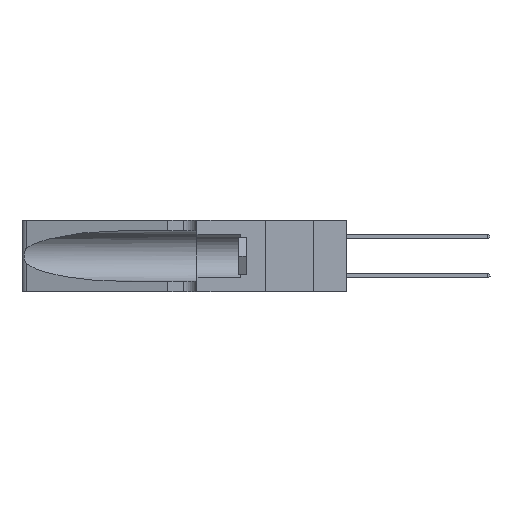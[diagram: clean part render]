
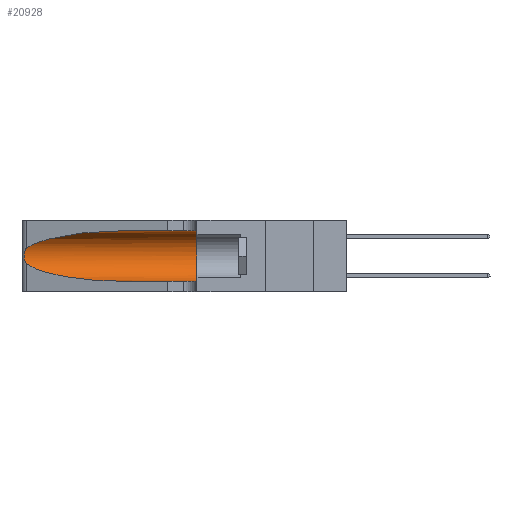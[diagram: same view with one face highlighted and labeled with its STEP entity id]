
A CAD part, left-side view. The second image highlights one B-rep face of the part: STEP entity #20928.
In plain terms, the highlighted cylindrical face has radius 3.308 mm (diameter 6.617 mm), a partial arc.
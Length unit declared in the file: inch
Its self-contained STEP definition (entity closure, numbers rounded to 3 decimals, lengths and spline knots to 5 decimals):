
#522 = VECTOR ( 'NONE', #25602, 39.37008 ) ;
#565 = AXIS2_PLACEMENT_3D ( 'NONE', #19608, #23783, #10734 ) ;
#960 = EDGE_CURVE ( 'NONE', #8144, #22175, #27132, .T. ) ;
#1241 = ORIENTED_EDGE ( 'NONE', *, *, #960, .T. ) ;
#1690 = VERTEX_POINT ( 'NONE', #23200 ) ;
#2027 = EDGE_LOOP ( 'NONE', ( #1241, #18153, #17085, #13312, #13359, #27412 ) ) ;
#2455 = EDGE_CURVE ( 'NONE', #8144, #1690, #9759, .T. ) ;
#3530 = EDGE_CURVE ( 'NONE', #1690, #6931, #11722, .T. ) ;
#3844 = DIRECTION ( 'NONE',  ( 0., 1., 0. ) ) ;
#4071 = CARTESIAN_POINT ( 'NONE',  ( 0.25487, 1.22718, 0.14631 ) ) ;
#4988 = FACE_OUTER_BOUND ( 'NONE', #2027, .T. ) ;
#5533 = CARTESIAN_POINT ( 'NONE',  ( 0.1305, 0.72297, 0.05475 ) ) ;
#6007 = CARTESIAN_POINT ( 'NONE',  ( 0.25854, 1.2359, 0.20912 ) ) ;
#6095 = CARTESIAN_POINT ( 'NONE',  ( 0.25639, 1.23184, 0.21858 ) ) ;
#6526 = CARTESIAN_POINT ( 'NONE',  ( 0.18966, 0.96281, 0.31525 ) ) ;
#6889 = VECTOR ( 'NONE', #8099, 39.37008 ) ;
#6931 = VERTEX_POINT ( 'NONE', #20959 ) ;
#7539 = CARTESIAN_POINT ( 'NONE',  ( 0.18966, 0.96281, 0.05475 ) ) ;
#8099 = DIRECTION ( 'NONE',  ( 0., -1., 0. ) ) ;
#8144 = VERTEX_POINT ( 'NONE', #23531 ) ;
#8605 = CARTESIAN_POINT ( 'NONE',  ( 0.26075, 1.23896, 0.19203 ) ) ;
#8644 = CARTESIAN_POINT ( 'NONE',  ( 0.25487, 1.22718, 0.14631 ) ) ;
#9153 = CARTESIAN_POINT ( 'NONE',  ( 0.25789, 1.23486, 0.15765 ) ) ;
#9521 = CARTESIAN_POINT ( 'NONE',  ( 0.2373, 1.15595, 0.08982 ) ) ;
#9759 = LINE ( 'NONE', #17137, #522 ) ;
#9943 = CARTESIAN_POINT ( 'NONE',  ( 0.25555, 1.22994, 0.2215 ) ) ;
#10236 = CARTESIAN_POINT ( 'NONE',  ( 0.26018, 1.23835, 0.19895 ) ) ;
#10396 = EDGE_CURVE ( 'NONE', #22175, #27143, #17878, .T. ) ;
#10734 = DIRECTION ( 'NONE',  ( 0., 0., -1. ) ) ;
#11075 = CARTESIAN_POINT ( 'NONE',  ( 0.26075, 1.23896, 0.178 ) ) ;
#11722 = CIRCLE ( 'NONE', #22953, 0.13025 ) ;
#13095 = CARTESIAN_POINT ( 'NONE',  ( 0.1305, 0.72297, 0.31525 ) ) ;
#13187 = CARTESIAN_POINT ( 'NONE',  ( 0.25487, 1.22718, 0.22369 ) ) ;
#13312 = ORIENTED_EDGE ( 'NONE', *, *, #27218, .T. ) ;
#13359 = ORIENTED_EDGE ( 'NONE', *, *, #3530, .F. ) ;
#13746 = EDGE_CURVE ( 'NONE', #27143, #21360, #19648, .T. ) ;
#14034 = CARTESIAN_POINT ( 'NONE',  ( 0.25487, 1.22718, 0.14631 ) ) ;
#15866 = CARTESIAN_POINT ( 'NONE',  ( 0.25487, 1.22718, 0.22369 ) ) ;
#16587 = CYLINDRICAL_SURFACE ( 'NONE', #565, 0.13025 ) ;
#17085 = ORIENTED_EDGE ( 'NONE', *, *, #13746, .T. ) ;
#17137 = CARTESIAN_POINT ( 'NONE',  ( 0.1305, 1.61858, 0.31525 ) ) ;
#17368 = CARTESIAN_POINT ( 'NONE',  ( 0.2373, 1.15595, 0.28018 ) ) ;
#17478 = CARTESIAN_POINT ( 'NONE',  ( 0.25639, 1.23186, 0.15144 ) ) ;
#17878 = B_SPLINE_CURVE_WITH_KNOTS ( 'NONE', 3,
 ( #26562, #9943, #6095, #23300, #6007, #10236, #8605, #11075, #27424, #23155, #9153, #17478, #21593, #8644 ),
 .UNSPECIFIED., .F., .F.,
 ( 4, 2, 2, 2, 2, 2, 4 ),
 ( 0., 0.00027, 0.00053, 0.00107, 0.0016, 0.00187, 0.00214 ),
 .UNSPECIFIED. ) ;
#18153 = ORIENTED_EDGE ( 'NONE', *, *, #10396, .T. ) ;
#19608 = CARTESIAN_POINT ( 'NONE',  ( 0.1305, 1.61858, 0.185 ) ) ;
#19648 =( BOUNDED_CURVE ( )  B_SPLINE_CURVE ( 3, ( #14034, #9521, #7539, #27119 ),
 .UNSPECIFIED., .F., .F. ) 
 B_SPLINE_CURVE_WITH_KNOTS ( ( 4, 4 ),
 ( 3.44316, 4.71239 ),
 .UNSPECIFIED. ) 
 CURVE ( )  GEOMETRIC_REPRESENTATION_ITEM ( )  RATIONAL_B_SPLINE_CURVE ( ( 1., 0.87, 0.87, 1. ) ) 
 REPRESENTATION_ITEM ( '' )  );
#20928 = ADVANCED_FACE ( 'NONE', ( #4988 ), #16587, .F. ) ;
#20959 = CARTESIAN_POINT ( 'NONE',  ( 0.1305, 0.35, 0.05475 ) ) ;
#21360 = VERTEX_POINT ( 'NONE', #5533 ) ;
#21386 = CARTESIAN_POINT ( 'NONE',  ( 0.1305, 0.35, 0.185 ) ) ;
#21593 = CARTESIAN_POINT ( 'NONE',  ( 0.25555, 1.22993, 0.14849 ) ) ;
#22175 = VERTEX_POINT ( 'NONE', #15866 ) ;
#22953 = AXIS2_PLACEMENT_3D ( 'NONE', #21386, #3844, #23568 ) ;
#23155 = CARTESIAN_POINT ( 'NONE',  ( 0.25856, 1.23593, 0.16098 ) ) ;
#23200 = CARTESIAN_POINT ( 'NONE',  ( 0.1305, 0.35, 0.31525 ) ) ;
#23300 = CARTESIAN_POINT ( 'NONE',  ( 0.25787, 1.23484, 0.2124 ) ) ;
#23531 = CARTESIAN_POINT ( 'NONE',  ( 0.1305, 0.72297, 0.31525 ) ) ;
#23568 = DIRECTION ( 'NONE',  ( 0., 0., 1. ) ) ;
#23783 = DIRECTION ( 'NONE',  ( 0., -1., 0. ) ) ;
#25394 = CARTESIAN_POINT ( 'NONE',  ( 0.1305, 1.61858, 0.05475 ) ) ;
#25602 = DIRECTION ( 'NONE',  ( 0., -1., 0. ) ) ;
#25947 = LINE ( 'NONE', #25394, #6889 ) ;
#26562 = CARTESIAN_POINT ( 'NONE',  ( 0.25487, 1.22718, 0.22369 ) ) ;
#27119 = CARTESIAN_POINT ( 'NONE',  ( 0.1305, 0.72297, 0.05475 ) ) ;
#27132 =( BOUNDED_CURVE ( )  B_SPLINE_CURVE ( 3, ( #13095, #6526, #17368, #13187 ),
 .UNSPECIFIED., .F., .T. ) 
 B_SPLINE_CURVE_WITH_KNOTS ( ( 4, 4 ),
 ( 1.5708, 2.84003 ),
 .UNSPECIFIED. ) 
 CURVE ( )  GEOMETRIC_REPRESENTATION_ITEM ( )  RATIONAL_B_SPLINE_CURVE ( ( 1., 0.87, 0.87, 1. ) ) 
 REPRESENTATION_ITEM ( '' )  );
#27143 = VERTEX_POINT ( 'NONE', #4071 ) ;
#27218 = EDGE_CURVE ( 'NONE', #21360, #6931, #25947, .T. ) ;
#27412 = ORIENTED_EDGE ( 'NONE', *, *, #2455, .F. ) ;
#27424 = CARTESIAN_POINT ( 'NONE',  ( 0.26017, 1.23833, 0.17102 ) ) ;
